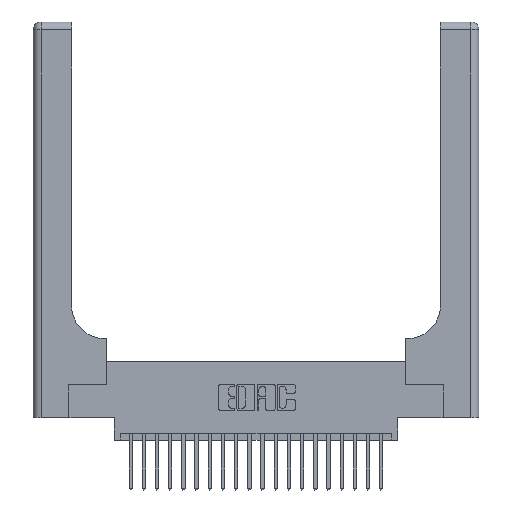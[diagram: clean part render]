
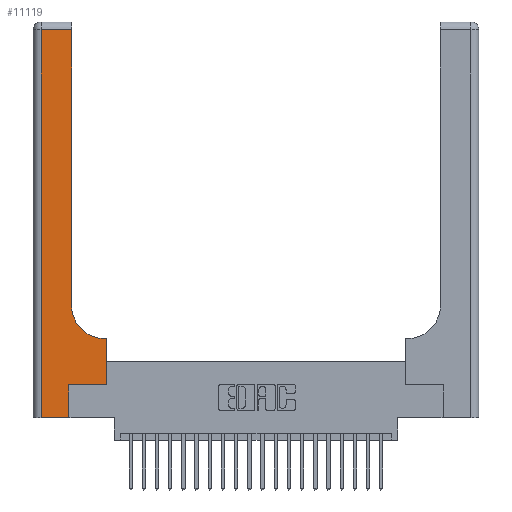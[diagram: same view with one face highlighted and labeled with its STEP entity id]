
A CAD part, top view. The second image highlights one B-rep face of the part: STEP entity #11119.
In plain terms, the highlighted planar face has unit normal (0, 0, 1).
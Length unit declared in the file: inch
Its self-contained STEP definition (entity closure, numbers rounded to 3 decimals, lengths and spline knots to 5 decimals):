
#193 = VERTEX_POINT ( 'NONE', #13688 ) ;
#595 = EDGE_CURVE ( 'NONE', #15929, #193, #1228, .T. ) ;
#721 = VECTOR ( 'NONE', #7281, 39.37008 ) ;
#816 = LINE ( 'NONE', #18812, #14753 ) ;
#865 = ORIENTED_EDGE ( 'NONE', *, *, #23380, .T. ) ;
#1126 = VECTOR ( 'NONE', #5600, 39.37008 ) ;
#1228 = LINE ( 'NONE', #7106, #5716 ) ;
#2507 = EDGE_CURVE ( 'NONE', #11055, #22771, #11271, .T. ) ;
#2637 = DIRECTION ( 'NONE',  ( 0., 1., 0. ) ) ;
#2777 = LINE ( 'NONE', #7901, #16021 ) ;
#2880 = LINE ( 'NONE', #19406, #7347 ) ;
#4357 = VECTOR ( 'NONE', #2637, 39.37008 ) ;
#4534 = EDGE_CURVE ( 'NONE', #8175, #8349, #2880, .T. ) ;
#4598 = CARTESIAN_POINT ( 'NONE',  ( 0.06, 2.94, 0.37 ) ) ;
#4718 = CARTESIAN_POINT ( 'NONE',  ( 0.5585, 0.25, 0.37 ) ) ;
#5353 = ORIENTED_EDGE ( 'NONE', *, *, #22841, .T. ) ;
#5600 = DIRECTION ( 'NONE',  ( 0., 1., 0. ) ) ;
#5716 = VECTOR ( 'NONE', #8134, 39.37008 ) ;
#5815 = LINE ( 'NONE', #9154, #721 ) ;
#6531 = ORIENTED_EDGE ( 'NONE', *, *, #9369, .T. ) ;
#7106 = CARTESIAN_POINT ( 'NONE',  ( 0.2915, 0.6, 0.37 ) ) ;
#7115 = VERTEX_POINT ( 'NONE', #4598 ) ;
#7130 = VERTEX_POINT ( 'NONE', #21335 ) ;
#7273 = AXIS2_PLACEMENT_3D ( 'NONE', #17224, #19052, #7987 ) ;
#7281 = DIRECTION ( 'NONE',  ( 1., 0., 0. ) ) ;
#7347 = VECTOR ( 'NONE', #21183, 39.37008 ) ;
#7820 = CARTESIAN_POINT ( 'NONE',  ( 0.2915, 0.85, 0.37 ) ) ;
#7901 = CARTESIAN_POINT ( 'NONE',  ( 0., 2.94, 0.37 ) ) ;
#7987 = DIRECTION ( 'NONE',  ( -1., 0., 0. ) ) ;
#8134 = DIRECTION ( 'NONE',  ( -1., 0., 0. ) ) ;
#8175 = VERTEX_POINT ( 'NONE', #20826 ) ;
#8349 = VERTEX_POINT ( 'NONE', #4718 ) ;
#8408 = CARTESIAN_POINT ( 'NONE',  ( 0.269, 0., 0.37 ) ) ;
#8621 = ORIENTED_EDGE ( 'NONE', *, *, #11108, .T. ) ;
#9154 = CARTESIAN_POINT ( 'NONE',  ( 0., 0., 0.37 ) ) ;
#9182 = CARTESIAN_POINT ( 'NONE',  ( 0.2915, 2.94, 0.37 ) ) ;
#9369 = EDGE_CURVE ( 'NONE', #21858, #8175, #9451, .T. ) ;
#9451 = LINE ( 'NONE', #12094, #4357 ) ;
#9637 = ORIENTED_EDGE ( 'NONE', *, *, #22681, .T. ) ;
#9673 = DIRECTION ( 'NONE',  ( 0., 1., 0. ) ) ;
#9940 = CARTESIAN_POINT ( 'NONE',  ( 0.5585, 0.6, 0.37 ) ) ;
#11055 = VERTEX_POINT ( 'NONE', #7820 ) ;
#11103 = FACE_OUTER_BOUND ( 'NONE', #18629, .T. ) ;
#11108 = EDGE_CURVE ( 'NONE', #22771, #7115, #2777, .T. ) ;
#11119 = ADVANCED_FACE ( 'NONE', ( #11103 ), #15407, .F. ) ;
#11271 = LINE ( 'NONE', #18613, #1126 ) ;
#11290 = CARTESIAN_POINT ( 'NONE',  ( 0.5415, 0.85, 0.37 ) ) ;
#11616 = DIRECTION ( 'NONE',  ( -1., 0., 0. ) ) ;
#11789 = VECTOR ( 'NONE', #14496, 39.37008 ) ;
#12094 = CARTESIAN_POINT ( 'NONE',  ( 0.269, 0., 0.37 ) ) ;
#13168 = DIRECTION ( 'NONE',  ( 1., 0., 0. ) ) ;
#13247 = CIRCLE ( 'NONE', #16713, 0.25 ) ;
#13688 = CARTESIAN_POINT ( 'NONE',  ( 0.5415, 0.6, 0.37 ) ) ;
#14422 = CARTESIAN_POINT ( 'NONE',  ( 0.06, 3., 0.37 ) ) ;
#14496 = DIRECTION ( 'NONE',  ( 0., -1., 0. ) ) ;
#14753 = VECTOR ( 'NONE', #9673, 39.37008 ) ;
#15407 = PLANE ( 'NONE',  #7273 ) ;
#15929 = VERTEX_POINT ( 'NONE', #9940 ) ;
#16021 = VECTOR ( 'NONE', #11616, 39.37008 ) ;
#16713 = AXIS2_PLACEMENT_3D ( 'NONE', #11290, #23920, #13168 ) ;
#16825 = ORIENTED_EDGE ( 'NONE', *, *, #595, .T. ) ;
#17224 = CARTESIAN_POINT ( 'NONE',  ( 0., 3., 0.37 ) ) ;
#17240 = LINE ( 'NONE', #14422, #11789 ) ;
#18613 = CARTESIAN_POINT ( 'NONE',  ( 0.2915, 3., 0.37 ) ) ;
#18629 = EDGE_LOOP ( 'NONE', ( #20611, #8621, #9637, #865, #6531, #20049, #19156, #16825, #5353 ) ) ;
#18812 = CARTESIAN_POINT ( 'NONE',  ( 0.5585, 0.25, 0.37 ) ) ;
#19052 = DIRECTION ( 'NONE',  ( 0., 0., -1. ) ) ;
#19156 = ORIENTED_EDGE ( 'NONE', *, *, #21622, .T. ) ;
#19406 = CARTESIAN_POINT ( 'NONE',  ( 0.269, 0.25, 0.37 ) ) ;
#20049 = ORIENTED_EDGE ( 'NONE', *, *, #4534, .T. ) ;
#20611 = ORIENTED_EDGE ( 'NONE', *, *, #2507, .T. ) ;
#20826 = CARTESIAN_POINT ( 'NONE',  ( 0.269, 0.25, 0.37 ) ) ;
#21183 = DIRECTION ( 'NONE',  ( 1., 0., 0. ) ) ;
#21335 = CARTESIAN_POINT ( 'NONE',  ( 0.06, 0., 0.37 ) ) ;
#21622 = EDGE_CURVE ( 'NONE', #8349, #15929, #816, .T. ) ;
#21858 = VERTEX_POINT ( 'NONE', #8408 ) ;
#22681 = EDGE_CURVE ( 'NONE', #7115, #7130, #17240, .T. ) ;
#22771 = VERTEX_POINT ( 'NONE', #9182 ) ;
#22841 = EDGE_CURVE ( 'NONE', #193, #11055, #13247, .T. ) ;
#23380 = EDGE_CURVE ( 'NONE', #7130, #21858, #5815, .T. ) ;
#23920 = DIRECTION ( 'NONE',  ( 0., 0., -1. ) ) ;
